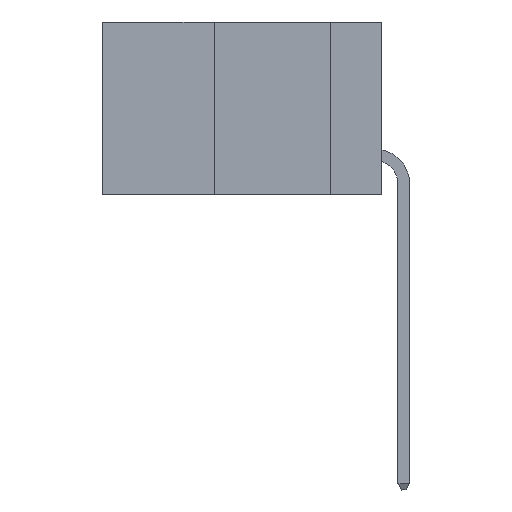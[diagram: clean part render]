
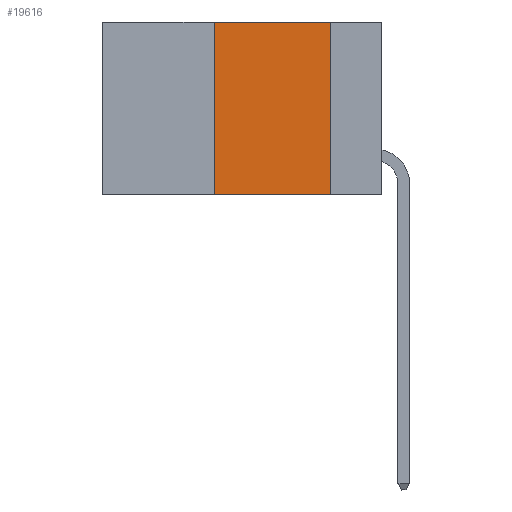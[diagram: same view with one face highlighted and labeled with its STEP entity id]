
A CAD part, left-side view. The second image highlights one B-rep face of the part: STEP entity #19616.
In plain terms, the highlighted planar face has unit normal (-1, 0, 0).
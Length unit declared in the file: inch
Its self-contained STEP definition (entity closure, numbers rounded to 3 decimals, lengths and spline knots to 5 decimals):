
#1236 = CARTESIAN_POINT ( 'NONE',  ( 0., 0.36, 0. ) ) ;
#1388 = VERTEX_POINT ( 'NONE', #2890 ) ;
#2404 = CARTESIAN_POINT ( 'NONE',  ( 0., 0.6, -0.37 ) ) ;
#2890 = CARTESIAN_POINT ( 'NONE',  ( 0., 0.36, -0.37 ) ) ;
#2961 = CARTESIAN_POINT ( 'NONE',  ( 0., 0.6, 0. ) ) ;
#3213 = ORIENTED_EDGE ( 'NONE', *, *, #16409, .F. ) ;
#3346 = VECTOR ( 'NONE', #15817, 39.37008 ) ;
#3573 = ORIENTED_EDGE ( 'NONE', *, *, #10866, .F. ) ;
#4110 = CARTESIAN_POINT ( 'NONE',  ( 0., 0.6, 0. ) ) ;
#5222 = LINE ( 'NONE', #17461, #23289 ) ;
#9039 = LINE ( 'NONE', #14347, #18723 ) ;
#9488 = EDGE_CURVE ( 'NONE', #1388, #15242, #18880, .T. ) ;
#9778 = DIRECTION ( 'NONE',  ( 0., 0., -1. ) ) ;
#10499 = VERTEX_POINT ( 'NONE', #1236 ) ;
#10866 = EDGE_CURVE ( 'NONE', #10499, #12756, #18508, .T. ) ;
#12756 = VERTEX_POINT ( 'NONE', #18364 ) ;
#12863 = ORIENTED_EDGE ( 'NONE', *, *, #23139, .F. ) ;
#13267 = DIRECTION ( 'NONE',  ( 0., 0., -1. ) ) ;
#14347 = CARTESIAN_POINT ( 'NONE',  ( 0., 0.36, 0. ) ) ;
#15242 = VERTEX_POINT ( 'NONE', #21463 ) ;
#15817 = DIRECTION ( 'NONE',  ( 0., -1., 0. ) ) ;
#16409 = EDGE_CURVE ( 'NONE', #12756, #15242, #5222, .T. ) ;
#16952 = DIRECTION ( 'NONE',  ( 1., 0., 0. ) ) ;
#17461 = CARTESIAN_POINT ( 'NONE',  ( 0., 0.11, 0. ) ) ;
#17982 = PLANE ( 'NONE',  #20764 ) ;
#18364 = CARTESIAN_POINT ( 'NONE',  ( 0., 0.11, 0. ) ) ;
#18434 = DIRECTION ( 'NONE',  ( 0., 0., 1. ) ) ;
#18508 = LINE ( 'NONE', #2961, #3346 ) ;
#18723 = VECTOR ( 'NONE', #18434, 39.37008 ) ;
#18765 = FACE_OUTER_BOUND ( 'NONE', #23285, .T. ) ;
#18880 = LINE ( 'NONE', #2404, #22043 ) ;
#18887 = DIRECTION ( 'NONE',  ( 0., -1., 0. ) ) ;
#19616 = ADVANCED_FACE ( 'NONE', ( #18765 ), #17982, .F. ) ;
#20764 = AXIS2_PLACEMENT_3D ( 'NONE', #4110, #16952, #13267 ) ;
#21463 = CARTESIAN_POINT ( 'NONE',  ( 0., 0.11, -0.37 ) ) ;
#22043 = VECTOR ( 'NONE', #18887, 39.37008 ) ;
#22491 = ORIENTED_EDGE ( 'NONE', *, *, #9488, .T. ) ;
#23139 = EDGE_CURVE ( 'NONE', #1388, #10499, #9039, .T. ) ;
#23285 = EDGE_LOOP ( 'NONE', ( #3213, #3573, #12863, #22491 ) ) ;
#23289 = VECTOR ( 'NONE', #9778, 39.37008 ) ;
